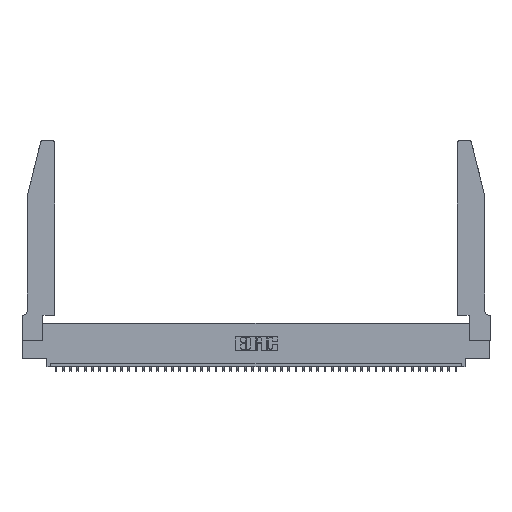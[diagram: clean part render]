
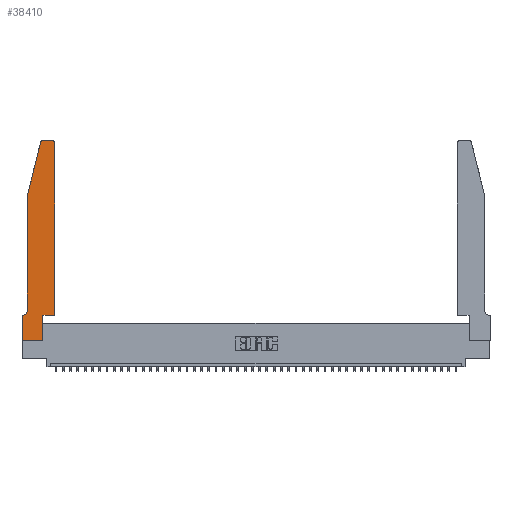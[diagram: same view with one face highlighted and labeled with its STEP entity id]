
A CAD part, top view. The second image highlights one B-rep face of the part: STEP entity #38410.
In plain terms, the highlighted planar face has unit normal (0, 0, 1).
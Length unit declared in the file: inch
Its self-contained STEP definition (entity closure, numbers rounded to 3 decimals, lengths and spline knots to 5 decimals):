
#57 = CARTESIAN_POINT ( 'NONE',  ( 0.2865, 0., 0.37 ) ) ;
#1103 = VECTOR ( 'NONE', #34738, 39.37008 ) ;
#1644 = EDGE_CURVE ( 'NONE', #26871, #3358, #15051, .T. ) ;
#2029 = VERTEX_POINT ( 'NONE', #5109 ) ;
#2281 = CARTESIAN_POINT ( 'NONE',  ( 0.284, 2.72, 0.37 ) ) ;
#2443 = DIRECTION ( 'NONE',  ( 1., 0., 0. ) ) ;
#2745 = ORIENTED_EDGE ( 'NONE', *, *, #23038, .T. ) ;
#2913 = CARTESIAN_POINT ( 'NONE',  ( 0.4505, 0.35, 0.37 ) ) ;
#3358 = VERTEX_POINT ( 'NONE', #5281 ) ;
#3708 = EDGE_CURVE ( 'NONE', #41766, #26871, #23099, .T. ) ;
#4606 = VERTEX_POINT ( 'NONE', #25336 ) ;
#5109 = CARTESIAN_POINT ( 'NONE',  ( 0.25487, 2.72718, 0.37 ) ) ;
#5135 = VERTEX_POINT ( 'NONE', #6815 ) ;
#5281 = CARTESIAN_POINT ( 'NONE',  ( 0.284, 2.75, 0.37 ) ) ;
#5557 = LINE ( 'NONE', #21199, #15337 ) ;
#6466 = CARTESIAN_POINT ( 'NONE',  ( 0.2865, 0.35, 0.37 ) ) ;
#6811 = CARTESIAN_POINT ( 'NONE',  ( 0.4205, 2.75, 0.37 ) ) ;
#6815 = CARTESIAN_POINT ( 'NONE',  ( 0., 0., 0.37 ) ) ;
#8473 = EDGE_CURVE ( 'NONE', #4606, #36869, #32386, .T. ) ;
#8893 = VECTOR ( 'NONE', #26454, 39.37008 ) ;
#9311 = CARTESIAN_POINT ( 'NONE',  ( 0., 0., 0.37 ) ) ;
#9751 = DIRECTION ( 'NONE',  ( 0., 0., 1. ) ) ;
#9921 = ORIENTED_EDGE ( 'NONE', *, *, #44329, .T. ) ;
#10472 = DIRECTION ( 'NONE',  ( 1., 0., 0. ) ) ;
#10539 = LINE ( 'NONE', #9311, #8893 ) ;
#10797 = CARTESIAN_POINT ( 'NONE',  ( 0.4205, 2.72, 0.37 ) ) ;
#10816 = ORIENTED_EDGE ( 'NONE', *, *, #19279, .T. ) ;
#11270 = DIRECTION ( 'NONE',  ( 1., 0., 0. ) ) ;
#12011 = DIRECTION ( 'NONE',  ( -0.239, -0.971, 0. ) ) ;
#12929 = ORIENTED_EDGE ( 'NONE', *, *, #13374, .T. ) ;
#13015 = CARTESIAN_POINT ( 'NONE',  ( 0.4505, 0.35, 0.37 ) ) ;
#13024 = ORIENTED_EDGE ( 'NONE', *, *, #33360, .T. ) ;
#13076 = LINE ( 'NONE', #6466, #33920 ) ;
#13374 = EDGE_CURVE ( 'NONE', #43354, #4606, #13076, .T. ) ;
#13406 = DIRECTION ( 'NONE',  ( -1., 0., 0. ) ) ;
#13746 = VERTEX_POINT ( 'NONE', #13973 ) ;
#13973 = CARTESIAN_POINT ( 'NONE',  ( 0.0755, 2., 0.37 ) ) ;
#14327 = DIRECTION ( 'NONE',  ( 1., 0., 0. ) ) ;
#14605 = ORIENTED_EDGE ( 'NONE', *, *, #39853, .T. ) ;
#15051 = LINE ( 'NONE', #41954, #23319 ) ;
#15088 = CARTESIAN_POINT ( 'NONE',  ( 0., 0., 0.37 ) ) ;
#15337 = VECTOR ( 'NONE', #28564, 39.37008 ) ;
#15620 = ORIENTED_EDGE ( 'NONE', *, *, #8473, .T. ) ;
#16250 = VERTEX_POINT ( 'NONE', #20828 ) ;
#16959 = DIRECTION ( 'NONE',  ( 0., 0., -1. ) ) ;
#17160 = ORIENTED_EDGE ( 'NONE', *, *, #38749, .T. ) ;
#17679 = EDGE_LOOP ( 'NONE', ( #24555, #9921, #14605, #35713, #13024, #2745, #17160, #40030, #12929, #15620, #10816, #35420 ) ) ;
#18137 = EDGE_CURVE ( 'NONE', #13746, #16250, #24682, .T. ) ;
#19279 = EDGE_CURVE ( 'NONE', #36869, #41766, #42223, .T. ) ;
#20828 = CARTESIAN_POINT ( 'NONE',  ( 0.0755, 0.42, 0.37 ) ) ;
#21199 = CARTESIAN_POINT ( 'NONE',  ( 0.0755, 0.35, 0.37 ) ) ;
#22041 = LINE ( 'NONE', #15088, #32475 ) ;
#23038 = EDGE_CURVE ( 'NONE', #28912, #25521, #5557, .T. ) ;
#23099 = CIRCLE ( 'NONE', #42104, 0.03 ) ;
#23319 = VECTOR ( 'NONE', #31851, 39.37008 ) ;
#24295 = CIRCLE ( 'NONE', #26239, 0.03 ) ;
#24555 = ORIENTED_EDGE ( 'NONE', *, *, #1644, .T. ) ;
#24682 = LINE ( 'NONE', #36595, #30753 ) ;
#25004 = AXIS2_PLACEMENT_3D ( 'NONE', #34406, #16959, #13406 ) ;
#25336 = CARTESIAN_POINT ( 'NONE',  ( 0.2865, 0.35, 0.37 ) ) ;
#25521 = VERTEX_POINT ( 'NONE', #39817 ) ;
#26239 = AXIS2_PLACEMENT_3D ( 'NONE', #2281, #9751, #2443 ) ;
#26454 = DIRECTION ( 'NONE',  ( 0., -1., 0. ) ) ;
#26871 = VERTEX_POINT ( 'NONE', #6811 ) ;
#28564 = DIRECTION ( 'NONE',  ( -1., 0., 0. ) ) ;
#28912 = VERTEX_POINT ( 'NONE', #41444 ) ;
#29035 = LINE ( 'NONE', #43018, #30154 ) ;
#30154 = VECTOR ( 'NONE', #12011, 39.37008 ) ;
#30180 = DIRECTION ( 'NONE',  ( 0., -1., 0. ) ) ;
#30280 = FACE_OUTER_BOUND ( 'NONE', #17679, .T. ) ;
#30460 = CARTESIAN_POINT ( 'NONE',  ( 0., 0.35, 0.37 ) ) ;
#30753 = VECTOR ( 'NONE', #30180, 39.37008 ) ;
#30835 = AXIS2_PLACEMENT_3D ( 'NONE', #30460, #33992, #44763 ) ;
#31851 = DIRECTION ( 'NONE',  ( -1., 0., 0. ) ) ;
#32386 = LINE ( 'NONE', #37398, #37326 ) ;
#32475 = VECTOR ( 'NONE', #11270, 39.37008 ) ;
#33360 = EDGE_CURVE ( 'NONE', #16250, #28912, #43863, .T. ) ;
#33920 = VECTOR ( 'NONE', #41655, 39.37008 ) ;
#33992 = DIRECTION ( 'NONE',  ( 0., 0., 1. ) ) ;
#34406 = CARTESIAN_POINT ( 'NONE',  ( 0.0055, 0.42, 0.37 ) ) ;
#34738 = DIRECTION ( 'NONE',  ( 0., 1., 0. ) ) ;
#35295 = DIRECTION ( 'NONE',  ( 0., 0., 1. ) ) ;
#35420 = ORIENTED_EDGE ( 'NONE', *, *, #3708, .T. ) ;
#35713 = ORIENTED_EDGE ( 'NONE', *, *, #18137, .T. ) ;
#35856 = CARTESIAN_POINT ( 'NONE',  ( 0.4505, 2.72, 0.37 ) ) ;
#36595 = CARTESIAN_POINT ( 'NONE',  ( 0.0755, 2., 0.37 ) ) ;
#36869 = VERTEX_POINT ( 'NONE', #13015 ) ;
#37326 = VECTOR ( 'NONE', #10472, 39.37008 ) ;
#37398 = CARTESIAN_POINT ( 'NONE',  ( 0.4505, 0.35, 0.37 ) ) ;
#38410 = ADVANCED_FACE ( 'NONE', ( #30280 ), #40700, .T. ) ;
#38749 = EDGE_CURVE ( 'NONE', #25521, #5135, #10539, .T. ) ;
#39817 = CARTESIAN_POINT ( 'NONE',  ( 0., 0.35, 0.37 ) ) ;
#39853 = EDGE_CURVE ( 'NONE', #2029, #13746, #29035, .T. ) ;
#40030 = ORIENTED_EDGE ( 'NONE', *, *, #44021, .T. ) ;
#40700 = PLANE ( 'NONE',  #30835 ) ;
#41444 = CARTESIAN_POINT ( 'NONE',  ( 0.0055, 0.35, 0.37 ) ) ;
#41655 = DIRECTION ( 'NONE',  ( 0., 1., 0. ) ) ;
#41766 = VERTEX_POINT ( 'NONE', #35856 ) ;
#41954 = CARTESIAN_POINT ( 'NONE',  ( 0.2605, 2.75, 0.37 ) ) ;
#42104 = AXIS2_PLACEMENT_3D ( 'NONE', #10797, #35295, #14327 ) ;
#42223 = LINE ( 'NONE', #2913, #1103 ) ;
#43018 = CARTESIAN_POINT ( 'NONE',  ( 0.0755, 2., 0.37 ) ) ;
#43354 = VERTEX_POINT ( 'NONE', #57 ) ;
#43863 = CIRCLE ( 'NONE', #25004, 0.07 ) ;
#44021 = EDGE_CURVE ( 'NONE', #5135, #43354, #22041, .T. ) ;
#44329 = EDGE_CURVE ( 'NONE', #3358, #2029, #24295, .T. ) ;
#44763 = DIRECTION ( 'NONE',  ( 1., 0., 0. ) ) ;
